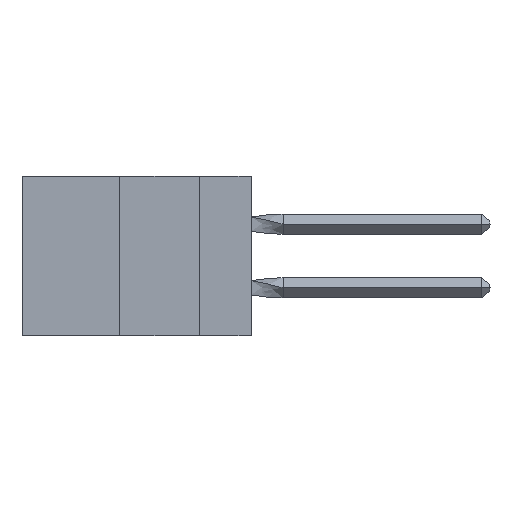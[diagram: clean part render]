
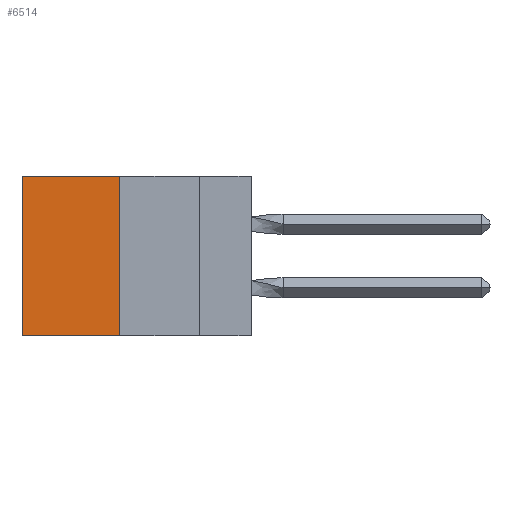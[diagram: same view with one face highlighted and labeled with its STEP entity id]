
A CAD part, left-side view. The second image highlights one B-rep face of the part: STEP entity #6514.
In plain terms, the highlighted planar face has unit normal (-1, 0, 0).
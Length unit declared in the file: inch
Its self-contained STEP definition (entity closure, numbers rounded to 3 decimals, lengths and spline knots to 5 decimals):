
#595 = DIRECTION ( 'NONE',  ( 0., 0., -1. ) ) ;
#728 = DIRECTION ( 'NONE',  ( 0., 1., 0. ) ) ;
#832 = DIRECTION ( 'NONE',  ( 0., 1., 0. ) ) ;
#2195 = ORIENTED_EDGE ( 'NONE', *, *, #8770, .F. ) ;
#2573 = DIRECTION ( 'NONE',  ( 0., 0., -1. ) ) ;
#2897 = VERTEX_POINT ( 'NONE', #6593 ) ;
#3253 = ORIENTED_EDGE ( 'NONE', *, *, #13893, .T. ) ;
#3705 = VECTOR ( 'NONE', #728, 39.37008 ) ;
#3762 = ORIENTED_EDGE ( 'NONE', *, *, #11774, .T. ) ;
#3959 = CARTESIAN_POINT ( 'NONE',  ( 0.305, 0.413, -0.5 ) ) ;
#4296 = VERTEX_POINT ( 'NONE', #7934 ) ;
#5022 = VECTOR ( 'NONE', #832, 39.37008 ) ;
#6303 = ORIENTED_EDGE ( 'NONE', *, *, #14701, .F. ) ;
#6425 = PLANE ( 'NONE',  #7195 ) ;
#6514 = ADVANCED_FACE ( 'NONE', ( #6643 ), #6425, .F. ) ;
#6593 = CARTESIAN_POINT ( 'NONE',  ( 0.305, 0.72, -0.5 ) ) ;
#6643 = FACE_OUTER_BOUND ( 'NONE', #7897, .T. ) ;
#6665 = VERTEX_POINT ( 'NONE', #6984 ) ;
#6803 = CARTESIAN_POINT ( 'NONE',  ( 0.305, 0.413, -0.5 ) ) ;
#6862 = DIRECTION ( 'NONE',  ( 0., 0., -1. ) ) ;
#6984 = CARTESIAN_POINT ( 'NONE',  ( 0.305, 0.413, 0. ) ) ;
#7125 = LINE ( 'NONE', #14523, #3705 ) ;
#7195 = AXIS2_PLACEMENT_3D ( 'NONE', #3959, #12236, #595 ) ;
#7897 = EDGE_LOOP ( 'NONE', ( #3762, #2195, #6303, #3253 ) ) ;
#7934 = CARTESIAN_POINT ( 'NONE',  ( 0.305, 0.72, 0. ) ) ;
#8636 = LINE ( 'NONE', #11689, #13871 ) ;
#8770 = EDGE_CURVE ( 'NONE', #12380, #2897, #7125, .T. ) ;
#9001 = LINE ( 'NONE', #6803, #14061 ) ;
#9816 = CARTESIAN_POINT ( 'NONE',  ( 0.305, 0.413, 0. ) ) ;
#10407 = CARTESIAN_POINT ( 'NONE',  ( 0.305, 0.413, -0.5 ) ) ;
#11689 = CARTESIAN_POINT ( 'NONE',  ( 0.305, 0.72, -0.5 ) ) ;
#11774 = EDGE_CURVE ( 'NONE', #4296, #2897, #8636, .T. ) ;
#12236 = DIRECTION ( 'NONE',  ( 1., 0., 0. ) ) ;
#12380 = VERTEX_POINT ( 'NONE', #10407 ) ;
#13871 = VECTOR ( 'NONE', #2573, 39.37008 ) ;
#13893 = EDGE_CURVE ( 'NONE', #6665, #4296, #14275, .T. ) ;
#14061 = VECTOR ( 'NONE', #6862, 39.37008 ) ;
#14275 = LINE ( 'NONE', #9816, #5022 ) ;
#14523 = CARTESIAN_POINT ( 'NONE',  ( 0.305, 0.413, -0.5 ) ) ;
#14701 = EDGE_CURVE ( 'NONE', #6665, #12380, #9001, .T. ) ;
